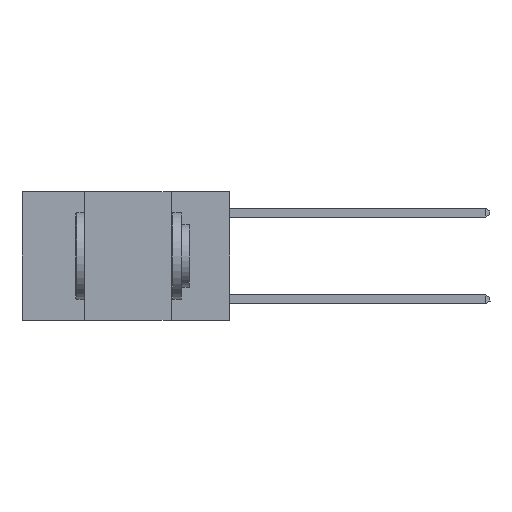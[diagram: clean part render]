
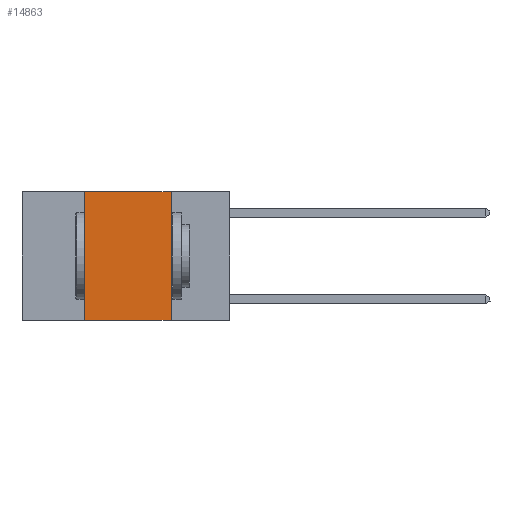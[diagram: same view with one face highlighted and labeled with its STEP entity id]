
A CAD part, left-side view. The second image highlights one B-rep face of the part: STEP entity #14863.
In plain terms, the highlighted planar face has unit normal (-1, 0, 0).
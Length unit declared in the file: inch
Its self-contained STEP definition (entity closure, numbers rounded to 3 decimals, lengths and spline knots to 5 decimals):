
#508 = CARTESIAN_POINT ( 'NONE',  ( 0., 0.6, 0. ) ) ;
#609 = CARTESIAN_POINT ( 'NONE',  ( 0., 0.42, 0. ) ) ;
#639 = ORIENTED_EDGE ( 'NONE', *, *, #5270, .T. ) ;
#759 = EDGE_LOOP ( 'NONE', ( #13280, #16768, #14118, #639 ) ) ;
#1391 = VERTEX_POINT ( 'NONE', #2663 ) ;
#1678 = CARTESIAN_POINT ( 'NONE',  ( 0., 0.17, -0.37 ) ) ;
#1802 = LINE ( 'NONE', #14214, #15615 ) ;
#2030 = LINE ( 'NONE', #10520, #15836 ) ;
#2663 = CARTESIAN_POINT ( 'NONE',  ( 0., 0.17, 0. ) ) ;
#3205 = CARTESIAN_POINT ( 'NONE',  ( 0., 0.42, 0. ) ) ;
#4640 = DIRECTION ( 'NONE',  ( 1., 0., 0. ) ) ;
#5162 = AXIS2_PLACEMENT_3D ( 'NONE', #508, #4640, #13985 ) ;
#5218 = DIRECTION ( 'NONE',  ( 0., -1., 0. ) ) ;
#5270 = EDGE_CURVE ( 'NONE', #14675, #10620, #11612, .T. ) ;
#6166 = EDGE_CURVE ( 'NONE', #14675, #9361, #16352, .T. ) ;
#6185 = VECTOR ( 'NONE', #8715, 39.37008 ) ;
#7515 = FACE_OUTER_BOUND ( 'NONE', #759, .T. ) ;
#8044 = DIRECTION ( 'NONE',  ( 0., -1., 0. ) ) ;
#8081 = VECTOR ( 'NONE', #8044, 39.37008 ) ;
#8715 = DIRECTION ( 'NONE',  ( 0., 0., 1. ) ) ;
#9361 = VERTEX_POINT ( 'NONE', #3205 ) ;
#10520 = CARTESIAN_POINT ( 'NONE',  ( 0., 0.6, 0. ) ) ;
#10620 = VERTEX_POINT ( 'NONE', #1678 ) ;
#11612 = LINE ( 'NONE', #12296, #8081 ) ;
#12224 = CARTESIAN_POINT ( 'NONE',  ( 0., 0.42, -0.37 ) ) ;
#12296 = CARTESIAN_POINT ( 'NONE',  ( 0., 0.6, -0.37 ) ) ;
#12945 = DIRECTION ( 'NONE',  ( 0., 0., -1. ) ) ;
#13280 = ORIENTED_EDGE ( 'NONE', *, *, #14985, .F. ) ;
#13586 = EDGE_CURVE ( 'NONE', #9361, #1391, #2030, .T. ) ;
#13926 = PLANE ( 'NONE',  #5162 ) ;
#13985 = DIRECTION ( 'NONE',  ( 0., 0., -1. ) ) ;
#14118 = ORIENTED_EDGE ( 'NONE', *, *, #6166, .F. ) ;
#14214 = CARTESIAN_POINT ( 'NONE',  ( 0., 0.17, 0. ) ) ;
#14675 = VERTEX_POINT ( 'NONE', #12224 ) ;
#14863 = ADVANCED_FACE ( 'NONE', ( #7515 ), #13926, .F. ) ;
#14985 = EDGE_CURVE ( 'NONE', #1391, #10620, #1802, .T. ) ;
#15615 = VECTOR ( 'NONE', #12945, 39.37008 ) ;
#15836 = VECTOR ( 'NONE', #5218, 39.37008 ) ;
#16352 = LINE ( 'NONE', #609, #6185 ) ;
#16768 = ORIENTED_EDGE ( 'NONE', *, *, #13586, .F. ) ;
